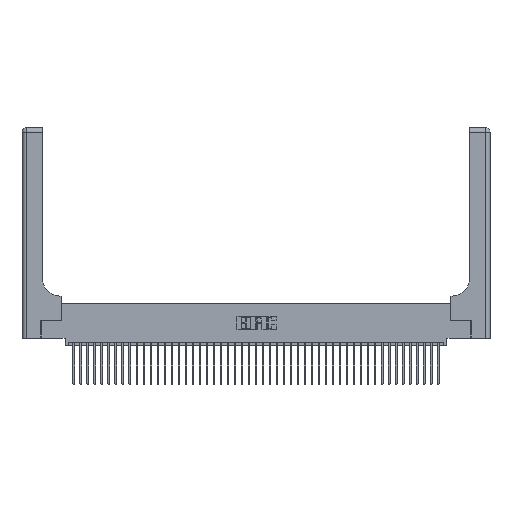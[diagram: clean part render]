
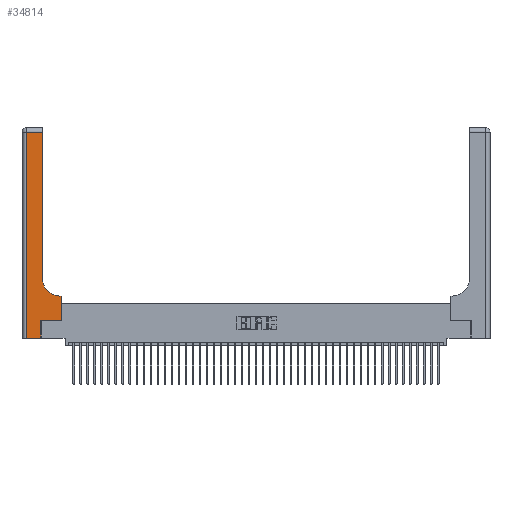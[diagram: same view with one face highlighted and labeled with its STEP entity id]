
A CAD part, top view. The second image highlights one B-rep face of the part: STEP entity #34814.
In plain terms, the highlighted planar face has unit normal (0, 0, 1).
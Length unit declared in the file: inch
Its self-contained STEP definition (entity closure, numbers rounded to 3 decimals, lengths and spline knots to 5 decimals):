
#1109 = VECTOR ( 'NONE', #19145, 39.37008 ) ;
#1623 = EDGE_CURVE ( 'NONE', #14693, #32964, #12784, .T. ) ;
#1635 = CARTESIAN_POINT ( 'NONE',  ( 0.2915, 0.6, 0.37 ) ) ;
#1805 = VECTOR ( 'NONE', #5516, 39.37008 ) ;
#2342 = VERTEX_POINT ( 'NONE', #41943 ) ;
#2723 = EDGE_CURVE ( 'NONE', #14741, #14046, #36809, .T. ) ;
#2828 = DIRECTION ( 'NONE',  ( 0., 0., -1. ) ) ;
#4877 = DIRECTION ( 'NONE',  ( -1., 0., 0. ) ) ;
#5467 = VECTOR ( 'NONE', #37371, 39.37008 ) ;
#5516 = DIRECTION ( 'NONE',  ( 0., 1., 0. ) ) ;
#6851 = EDGE_CURVE ( 'NONE', #12855, #2342, #31859, .T. ) ;
#7693 = CARTESIAN_POINT ( 'NONE',  ( 0.06, 0., 0.37 ) ) ;
#8220 = ORIENTED_EDGE ( 'NONE', *, *, #21783, .T. ) ;
#8278 = EDGE_CURVE ( 'NONE', #35681, #39308, #37731, .T. ) ;
#8352 = EDGE_LOOP ( 'NONE', ( #37389, #16486, #16284, #31715, #33063, #8220, #44545, #29821, #20371 ) ) ;
#8514 = DIRECTION ( 'NONE',  ( 0., 0., -1. ) ) ;
#9827 = CIRCLE ( 'NONE', #37782, 0.25 ) ;
#11011 = VECTOR ( 'NONE', #11235, 39.37008 ) ;
#11235 = DIRECTION ( 'NONE',  ( 0., -1., 0. ) ) ;
#11480 = VECTOR ( 'NONE', #4877, 39.37008 ) ;
#12479 = PLANE ( 'NONE',  #27523 ) ;
#12784 = LINE ( 'NONE', #23045, #1805 ) ;
#12803 = EDGE_CURVE ( 'NONE', #2342, #14693, #9827, .T. ) ;
#12855 = VERTEX_POINT ( 'NONE', #14612 ) ;
#13723 = CARTESIAN_POINT ( 'NONE',  ( 0., 2.94, 0.37 ) ) ;
#14046 = VERTEX_POINT ( 'NONE', #7693 ) ;
#14317 = CARTESIAN_POINT ( 'NONE',  ( 0.06, 2.94, 0.37 ) ) ;
#14612 = CARTESIAN_POINT ( 'NONE',  ( 0.5585, 0.6, 0.37 ) ) ;
#14693 = VERTEX_POINT ( 'NONE', #39374 ) ;
#14733 = FACE_OUTER_BOUND ( 'NONE', #8352, .T. ) ;
#14741 = VERTEX_POINT ( 'NONE', #14317 ) ;
#16284 = ORIENTED_EDGE ( 'NONE', *, *, #2723, .T. ) ;
#16486 = ORIENTED_EDGE ( 'NONE', *, *, #36046, .T. ) ;
#17146 = LINE ( 'NONE', #33077, #38479 ) ;
#19145 = DIRECTION ( 'NONE',  ( 1., 0., 0. ) ) ;
#20371 = ORIENTED_EDGE ( 'NONE', *, *, #12803, .T. ) ;
#20963 = DIRECTION ( 'NONE',  ( -1., 0., 0. ) ) ;
#21184 = VERTEX_POINT ( 'NONE', #32575 ) ;
#21516 = LINE ( 'NONE', #36701, #1109 ) ;
#21783 = EDGE_CURVE ( 'NONE', #39308, #21184, #17146, .T. ) ;
#23045 = CARTESIAN_POINT ( 'NONE',  ( 0.2915, 3., 0.37 ) ) ;
#23307 = EDGE_CURVE ( 'NONE', #21184, #12855, #31252, .T. ) ;
#25155 = VECTOR ( 'NONE', #43489, 39.37008 ) ;
#26231 = CARTESIAN_POINT ( 'NONE',  ( 0.5415, 0.85, 0.37 ) ) ;
#26249 = CARTESIAN_POINT ( 'NONE',  ( 0.2915, 2.94, 0.37 ) ) ;
#26654 = DIRECTION ( 'NONE',  ( -1., 0., 0. ) ) ;
#26725 = VECTOR ( 'NONE', #20963, 39.37008 ) ;
#27523 = AXIS2_PLACEMENT_3D ( 'NONE', #39930, #8514, #26654 ) ;
#27821 = CARTESIAN_POINT ( 'NONE',  ( 0.269, 0.25, 0.37 ) ) ;
#28072 = EDGE_CURVE ( 'NONE', #14046, #35681, #21516, .T. ) ;
#28423 = CARTESIAN_POINT ( 'NONE',  ( 0.5585, 0.25, 0.37 ) ) ;
#29821 = ORIENTED_EDGE ( 'NONE', *, *, #6851, .T. ) ;
#31252 = LINE ( 'NONE', #28423, #5467 ) ;
#31715 = ORIENTED_EDGE ( 'NONE', *, *, #28072, .T. ) ;
#31859 = LINE ( 'NONE', #1635, #11480 ) ;
#32575 = CARTESIAN_POINT ( 'NONE',  ( 0.5585, 0.25, 0.37 ) ) ;
#32964 = VERTEX_POINT ( 'NONE', #26249 ) ;
#33063 = ORIENTED_EDGE ( 'NONE', *, *, #8278, .T. ) ;
#33077 = CARTESIAN_POINT ( 'NONE',  ( 0.269, 0.25, 0.37 ) ) ;
#33789 = LINE ( 'NONE', #13723, #26725 ) ;
#34814 = ADVANCED_FACE ( 'NONE', ( #14733 ), #12479, .F. ) ;
#35681 = VERTEX_POINT ( 'NONE', #45426 ) ;
#35825 = DIRECTION ( 'NONE',  ( 1., 0., 0. ) ) ;
#36046 = EDGE_CURVE ( 'NONE', #32964, #14741, #33789, .T. ) ;
#36701 = CARTESIAN_POINT ( 'NONE',  ( 0., 0., 0.37 ) ) ;
#36809 = LINE ( 'NONE', #37090, #11011 ) ;
#37090 = CARTESIAN_POINT ( 'NONE',  ( 0.06, 3., 0.37 ) ) ;
#37371 = DIRECTION ( 'NONE',  ( 0., 1., 0. ) ) ;
#37389 = ORIENTED_EDGE ( 'NONE', *, *, #1623, .T. ) ;
#37731 = LINE ( 'NONE', #43008, #25155 ) ;
#37782 = AXIS2_PLACEMENT_3D ( 'NONE', #26231, #2828, #41653 ) ;
#38479 = VECTOR ( 'NONE', #35825, 39.37008 ) ;
#39308 = VERTEX_POINT ( 'NONE', #27821 ) ;
#39374 = CARTESIAN_POINT ( 'NONE',  ( 0.2915, 0.85, 0.37 ) ) ;
#39930 = CARTESIAN_POINT ( 'NONE',  ( 0., 3., 0.37 ) ) ;
#41653 = DIRECTION ( 'NONE',  ( 1., 0., 0. ) ) ;
#41943 = CARTESIAN_POINT ( 'NONE',  ( 0.5415, 0.6, 0.37 ) ) ;
#43008 = CARTESIAN_POINT ( 'NONE',  ( 0.269, 0., 0.37 ) ) ;
#43489 = DIRECTION ( 'NONE',  ( 0., 1., 0. ) ) ;
#44545 = ORIENTED_EDGE ( 'NONE', *, *, #23307, .T. ) ;
#45426 = CARTESIAN_POINT ( 'NONE',  ( 0.269, 0., 0.37 ) ) ;
